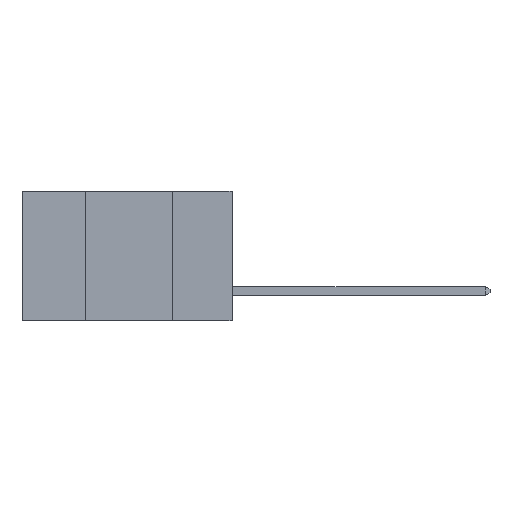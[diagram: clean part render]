
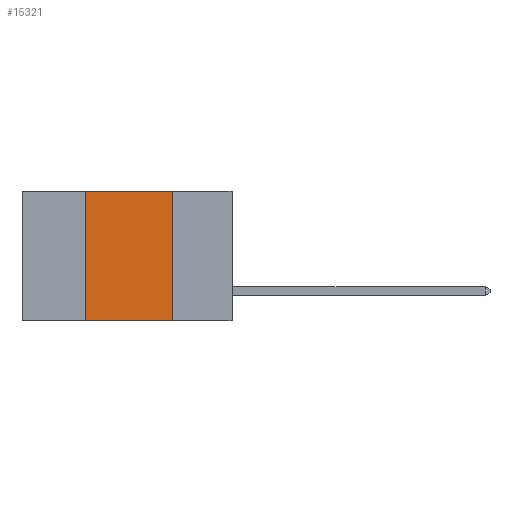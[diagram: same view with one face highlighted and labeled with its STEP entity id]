
A CAD part, left-side view. The second image highlights one B-rep face of the part: STEP entity #15321.
In plain terms, the highlighted planar face has unit normal (-1, 0, 0).
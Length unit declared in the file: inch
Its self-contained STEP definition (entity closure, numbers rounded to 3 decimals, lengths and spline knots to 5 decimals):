
#480 = AXIS2_PLACEMENT_3D ( 'NONE', #1658, #24099, #4897 ) ;
#1658 = CARTESIAN_POINT ( 'NONE',  ( 0., 0.6, 0. ) ) ;
#2239 = VECTOR ( 'NONE', #17011, 39.37008 ) ;
#4897 = DIRECTION ( 'NONE',  ( 0., 0., -1. ) ) ;
#6870 = VERTEX_POINT ( 'NONE', #19399 ) ;
#7220 = CARTESIAN_POINT ( 'NONE',  ( 0., 0.42, 0. ) ) ;
#8137 = PLANE ( 'NONE',  #480 ) ;
#9488 = VECTOR ( 'NONE', #27784, 39.37008 ) ;
#9581 = CARTESIAN_POINT ( 'NONE',  ( 0., 0.6, -0.37 ) ) ;
#10778 = LINE ( 'NONE', #29537, #2239 ) ;
#10866 = DIRECTION ( 'NONE',  ( 0., 0., 1. ) ) ;
#11999 = LINE ( 'NONE', #27915, #9488 ) ;
#15321 = ADVANCED_FACE ( 'NONE', ( #36239 ), #8137, .F. ) ;
#17011 = DIRECTION ( 'NONE',  ( 0., -1., 0. ) ) ;
#17174 = CARTESIAN_POINT ( 'NONE',  ( 0., 0.17, -0.37 ) ) ;
#17706 = CARTESIAN_POINT ( 'NONE',  ( 0., 0.42, 0. ) ) ;
#17884 = ORIENTED_EDGE ( 'NONE', *, *, #28440, .F. ) ;
#19399 = CARTESIAN_POINT ( 'NONE',  ( 0., 0.17, 0. ) ) ;
#20399 = EDGE_LOOP ( 'NONE', ( #36492, #28566, #17884, #23123 ) ) ;
#20506 = EDGE_CURVE ( 'NONE', #6870, #39922, #11999, .T. ) ;
#20592 = VERTEX_POINT ( 'NONE', #31659 ) ;
#22188 = VERTEX_POINT ( 'NONE', #17706 ) ;
#23094 = EDGE_CURVE ( 'NONE', #20592, #39922, #29244, .T. ) ;
#23123 = ORIENTED_EDGE ( 'NONE', *, *, #23094, .T. ) ;
#24099 = DIRECTION ( 'NONE',  ( 1., 0., 0. ) ) ;
#27784 = DIRECTION ( 'NONE',  ( 0., 0., -1. ) ) ;
#27915 = CARTESIAN_POINT ( 'NONE',  ( 0., 0.17, 0. ) ) ;
#28440 = EDGE_CURVE ( 'NONE', #20592, #22188, #29112, .T. ) ;
#28566 = ORIENTED_EDGE ( 'NONE', *, *, #32398, .F. ) ;
#29112 = LINE ( 'NONE', #7220, #30098 ) ;
#29244 = LINE ( 'NONE', #9581, #30250 ) ;
#29537 = CARTESIAN_POINT ( 'NONE',  ( 0., 0.6, 0. ) ) ;
#30098 = VECTOR ( 'NONE', #10866, 39.37008 ) ;
#30250 = VECTOR ( 'NONE', #41261, 39.37008 ) ;
#31659 = CARTESIAN_POINT ( 'NONE',  ( 0., 0.42, -0.37 ) ) ;
#32398 = EDGE_CURVE ( 'NONE', #22188, #6870, #10778, .T. ) ;
#36239 = FACE_OUTER_BOUND ( 'NONE', #20399, .T. ) ;
#36492 = ORIENTED_EDGE ( 'NONE', *, *, #20506, .F. ) ;
#39922 = VERTEX_POINT ( 'NONE', #17174 ) ;
#41261 = DIRECTION ( 'NONE',  ( 0., -1., 0. ) ) ;
